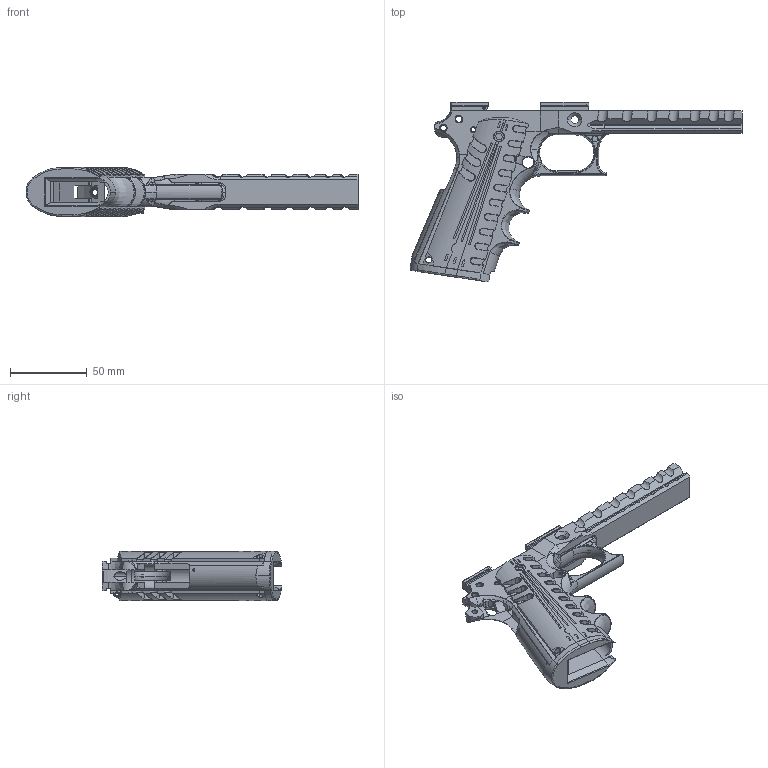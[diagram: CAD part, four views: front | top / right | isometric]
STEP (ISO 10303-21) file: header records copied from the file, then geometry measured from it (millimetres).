
FILE_DESCRIPTION (( 'STEP AP214' ), '1' );
FILE_NAME ('1911_2 teiliges Griffstück.STEP', '2013-07-30T15:10:44', ( 'Asher' ), ( '' ), 'SwSTEP 2.0', 'SolidWorks 2013', '' );
FILE_SCHEMA (( 'AUTOMOTIVE_DESIGN' ));
Length unit declared in the file: millimetre
Products named in the file (7): 4.04mm_Stift_Standard; 5503841; Zentrierstück; Schraube_Griffstück; Grip_Single; Frame_Single_Tactical_5Zoll; 1911_2 teiliges Griffstück
Assembly tree (8 placements, depth 2):
  1911_2 teiliges Griffstück
    Frame_Single_Tactical_5Zoll
    Grip_Single
    Schraube_Griffstück  x2
    Zentrierstück  x2
    5503841
    4.04mm_Stift_Standard
Bounding box: 216.3 x 116.93 x 32.11 mm (x, y, z)
Volume: 104217.4 mm3; surface area: 61775.9 mm2
Topology: 8 solids, 10 shells, 1438 faces, 3886 edges, 2475 vertices
Faces by surface type: plane 542, cylinder 513, bspline 227, cone 76, torus 76, sphere 4
Entity records: 54744 total; most frequent: CARTESIAN_POINT 22732, ORIENTED_EDGE 7272, DIRECTION 5646, EDGE_CURVE 3636, VERTEX_POINT 2321, AXIS2_PLACEMENT_3D 1995, VECTOR 1656, LINE 1656
